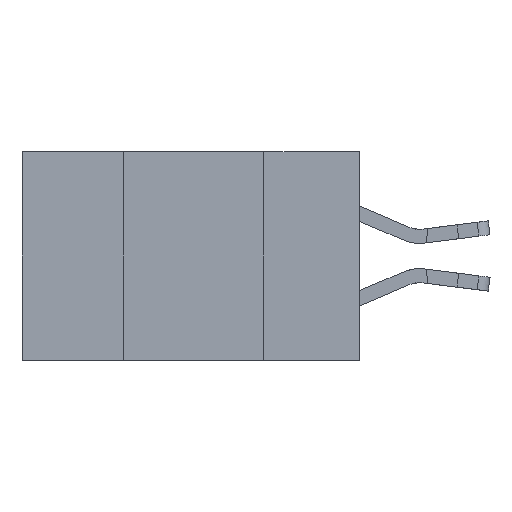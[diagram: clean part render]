
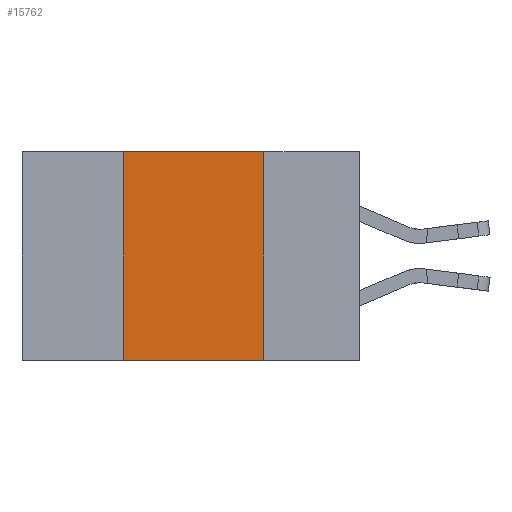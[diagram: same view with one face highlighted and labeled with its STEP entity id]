
A CAD part, left-side view. The second image highlights one B-rep face of the part: STEP entity #15762.
In plain terms, the highlighted planar face has unit normal (-1, 0, 0).
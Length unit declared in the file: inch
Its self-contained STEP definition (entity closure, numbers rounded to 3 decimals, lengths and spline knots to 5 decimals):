
#610 = CARTESIAN_POINT ( 'NONE',  ( 0., 0.17, 0. ) ) ;
#1656 = ORIENTED_EDGE ( 'NONE', *, *, #4389, .F. ) ;
#2140 = DIRECTION ( 'NONE',  ( 0., 0., -1. ) ) ;
#2553 = EDGE_CURVE ( 'NONE', #5065, #5438, #10061, .T. ) ;
#2969 = VERTEX_POINT ( 'NONE', #3653 ) ;
#3613 = LINE ( 'NONE', #17410, #11394 ) ;
#3653 = CARTESIAN_POINT ( 'NONE',  ( 0., 0.17, -0.37 ) ) ;
#4389 = EDGE_CURVE ( 'NONE', #5438, #8815, #15835, .T. ) ;
#5065 = VERTEX_POINT ( 'NONE', #14911 ) ;
#5435 = ORIENTED_EDGE ( 'NONE', *, *, #2553, .F. ) ;
#5438 = VERTEX_POINT ( 'NONE', #19702 ) ;
#5909 = VECTOR ( 'NONE', #10727, 39.37008 ) ;
#6026 = ORIENTED_EDGE ( 'NONE', *, *, #17431, .T. ) ;
#8546 = ORIENTED_EDGE ( 'NONE', *, *, #8647, .F. ) ;
#8647 = EDGE_CURVE ( 'NONE', #8815, #2969, #13081, .T. ) ;
#8658 = VECTOR ( 'NONE', #10383, 39.37008 ) ;
#8815 = VERTEX_POINT ( 'NONE', #14770 ) ;
#9078 = CARTESIAN_POINT ( 'NONE',  ( 0., 0.6, 0. ) ) ;
#10061 = LINE ( 'NONE', #17725, #5909 ) ;
#10383 = DIRECTION ( 'NONE',  ( 0., -1., 0. ) ) ;
#10637 = DIRECTION ( 'NONE',  ( 0., 0., -1. ) ) ;
#10727 = DIRECTION ( 'NONE',  ( 0., 0., 1. ) ) ;
#10784 = FACE_OUTER_BOUND ( 'NONE', #15799, .T. ) ;
#11394 = VECTOR ( 'NONE', #18927, 39.37008 ) ;
#13081 = LINE ( 'NONE', #610, #16635 ) ;
#14770 = CARTESIAN_POINT ( 'NONE',  ( 0., 0.17, 0. ) ) ;
#14911 = CARTESIAN_POINT ( 'NONE',  ( 0., 0.42, -0.37 ) ) ;
#15762 = ADVANCED_FACE ( 'NONE', ( #10784 ), #16685, .F. ) ;
#15799 = EDGE_LOOP ( 'NONE', ( #8546, #1656, #5435, #6026 ) ) ;
#15835 = LINE ( 'NONE', #16847, #8658 ) ;
#16635 = VECTOR ( 'NONE', #2140, 39.37008 ) ;
#16685 = PLANE ( 'NONE',  #19521 ) ;
#16847 = CARTESIAN_POINT ( 'NONE',  ( 0., 0.6, 0. ) ) ;
#17410 = CARTESIAN_POINT ( 'NONE',  ( 0., 0.6, -0.37 ) ) ;
#17431 = EDGE_CURVE ( 'NONE', #5065, #2969, #3613, .T. ) ;
#17725 = CARTESIAN_POINT ( 'NONE',  ( 0., 0.42, 0. ) ) ;
#18927 = DIRECTION ( 'NONE',  ( 0., -1., 0. ) ) ;
#19521 = AXIS2_PLACEMENT_3D ( 'NONE', #9078, #19709, #10637 ) ;
#19702 = CARTESIAN_POINT ( 'NONE',  ( 0., 0.42, 0. ) ) ;
#19709 = DIRECTION ( 'NONE',  ( 1., 0., 0. ) ) ;
